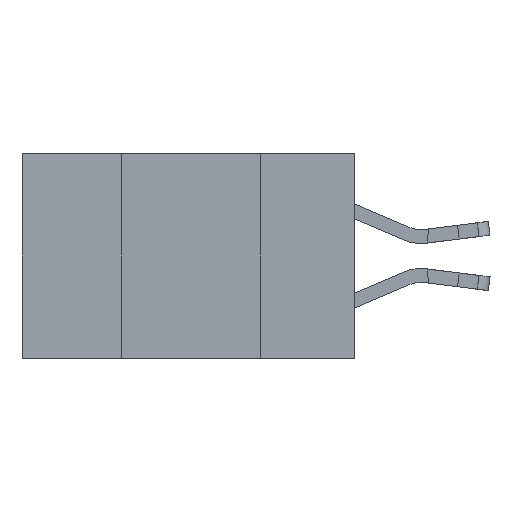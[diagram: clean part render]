
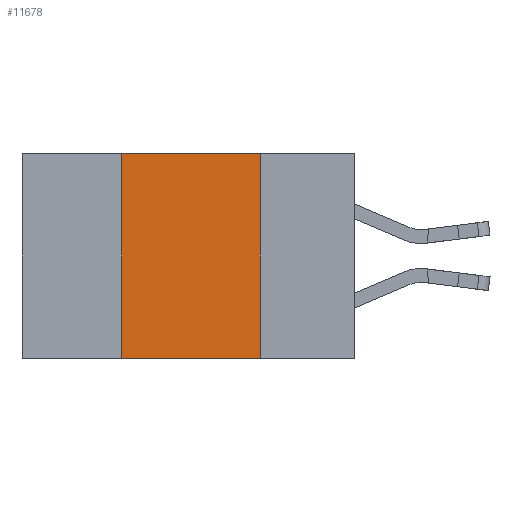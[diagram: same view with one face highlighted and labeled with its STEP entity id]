
A CAD part, left-side view. The second image highlights one B-rep face of the part: STEP entity #11678.
In plain terms, the highlighted planar face has unit normal (-1, 0, 0).
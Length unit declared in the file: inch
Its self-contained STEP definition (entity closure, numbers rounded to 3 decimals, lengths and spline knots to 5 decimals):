
#946 = VERTEX_POINT ( 'NONE', #20125 ) ;
#1228 = DIRECTION ( 'NONE',  ( 0., 0., -1. ) ) ;
#2429 = EDGE_CURVE ( 'NONE', #14412, #15661, #10893, .T. ) ;
#2886 = ORIENTED_EDGE ( 'NONE', *, *, #10105, .F. ) ;
#4374 = DIRECTION ( 'NONE',  ( 0., -1., 0. ) ) ;
#5167 = DIRECTION ( 'NONE',  ( 0., -1., 0. ) ) ;
#6760 = LINE ( 'NONE', #21341, #11726 ) ;
#7260 = LINE ( 'NONE', #10580, #18588 ) ;
#7897 = CARTESIAN_POINT ( 'NONE',  ( 0., 0.6, 0. ) ) ;
#9479 = LINE ( 'NONE', #16570, #18720 ) ;
#9725 = CARTESIAN_POINT ( 'NONE',  ( 0., 0.17, -0.37 ) ) ;
#10096 = VERTEX_POINT ( 'NONE', #15845 ) ;
#10105 = EDGE_CURVE ( 'NONE', #14412, #946, #9479, .T. ) ;
#10580 = CARTESIAN_POINT ( 'NONE',  ( 0., 0.6, 0. ) ) ;
#10893 = LINE ( 'NONE', #19855, #15779 ) ;
#11114 = DIRECTION ( 'NONE',  ( 1., 0., 0. ) ) ;
#11646 = DIRECTION ( 'NONE',  ( 0., 0., 1. ) ) ;
#11678 = ADVANCED_FACE ( 'NONE', ( #13771 ), #12780, .F. ) ;
#11726 = VECTOR ( 'NONE', #13160, 39.37008 ) ;
#11809 = AXIS2_PLACEMENT_3D ( 'NONE', #7897, #11114, #1228 ) ;
#12780 = PLANE ( 'NONE',  #11809 ) ;
#13160 = DIRECTION ( 'NONE',  ( 0., 0., -1. ) ) ;
#13758 = EDGE_CURVE ( 'NONE', #946, #10096, #7260, .T. ) ;
#13771 = FACE_OUTER_BOUND ( 'NONE', #14938, .T. ) ;
#14412 = VERTEX_POINT ( 'NONE', #18410 ) ;
#14938 = EDGE_LOOP ( 'NONE', ( #18808, #21397, #2886, #16409 ) ) ;
#15002 = EDGE_CURVE ( 'NONE', #10096, #15661, #6760, .T. ) ;
#15661 = VERTEX_POINT ( 'NONE', #9725 ) ;
#15779 = VECTOR ( 'NONE', #5167, 39.37008 ) ;
#15845 = CARTESIAN_POINT ( 'NONE',  ( 0., 0.17, 0. ) ) ;
#16409 = ORIENTED_EDGE ( 'NONE', *, *, #2429, .T. ) ;
#16570 = CARTESIAN_POINT ( 'NONE',  ( 0., 0.42, 0. ) ) ;
#18410 = CARTESIAN_POINT ( 'NONE',  ( 0., 0.42, -0.37 ) ) ;
#18588 = VECTOR ( 'NONE', #4374, 39.37008 ) ;
#18720 = VECTOR ( 'NONE', #11646, 39.37008 ) ;
#18808 = ORIENTED_EDGE ( 'NONE', *, *, #15002, .F. ) ;
#19855 = CARTESIAN_POINT ( 'NONE',  ( 0., 0.6, -0.37 ) ) ;
#20125 = CARTESIAN_POINT ( 'NONE',  ( 0., 0.42, 0. ) ) ;
#21341 = CARTESIAN_POINT ( 'NONE',  ( 0., 0.17, 0. ) ) ;
#21397 = ORIENTED_EDGE ( 'NONE', *, *, #13758, .F. ) ;
